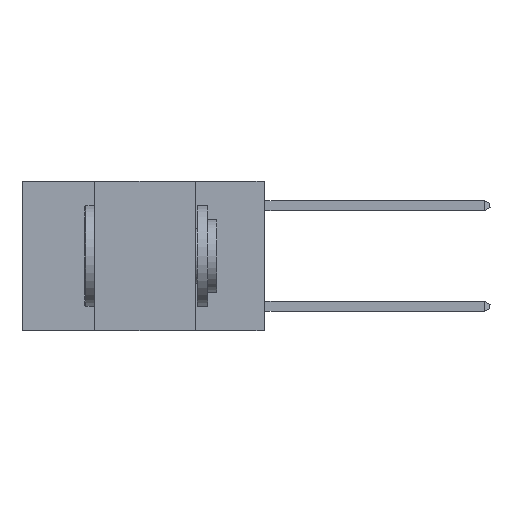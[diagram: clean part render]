
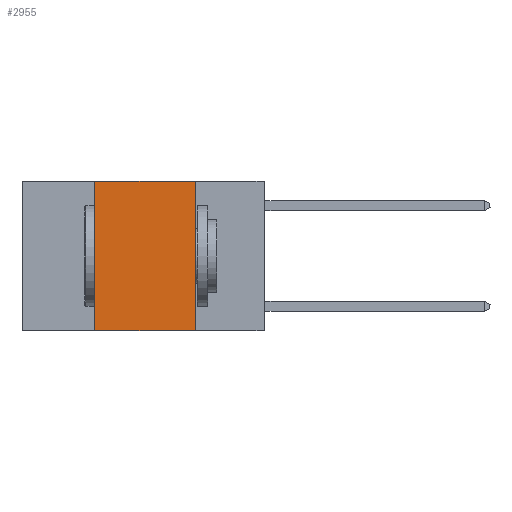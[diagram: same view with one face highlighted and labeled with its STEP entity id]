
A CAD part, left-side view. The second image highlights one B-rep face of the part: STEP entity #2955.
In plain terms, the highlighted planar face has unit normal (-1, 0, 0).
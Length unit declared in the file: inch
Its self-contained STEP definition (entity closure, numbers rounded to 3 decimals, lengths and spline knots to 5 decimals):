
#1292 = ORIENTED_EDGE ( 'NONE', *, *, #1631, .T. ) ;
#1631 = EDGE_CURVE ( 'NONE', #12407, #27223, #18043, .T. ) ;
#1664 = CARTESIAN_POINT ( 'NONE',  ( 0., 0.17, -0.37 ) ) ;
#2785 = ORIENTED_EDGE ( 'NONE', *, *, #22807, .F. ) ;
#2955 = ADVANCED_FACE ( 'NONE', ( #5064 ), #23852, .F. ) ;
#3249 = CARTESIAN_POINT ( 'NONE',  ( 0., 0.42, 0. ) ) ;
#3257 = LINE ( 'NONE', #19297, #18643 ) ;
#3415 = ORIENTED_EDGE ( 'NONE', *, *, #21486, .F. ) ;
#4548 = VERTEX_POINT ( 'NONE', #15883 ) ;
#4692 = CARTESIAN_POINT ( 'NONE',  ( 0., 0.6, 0. ) ) ;
#5050 = EDGE_CURVE ( 'NONE', #4548, #10568, #18582, .T. ) ;
#5064 = FACE_OUTER_BOUND ( 'NONE', #8661, .T. ) ;
#5957 = VECTOR ( 'NONE', #13002, 39.37008 ) ;
#6549 = DIRECTION ( 'NONE',  ( 0., -1., 0. ) ) ;
#7078 = ORIENTED_EDGE ( 'NONE', *, *, #5050, .F. ) ;
#8661 = EDGE_LOOP ( 'NONE', ( #2785, #7078, #3415, #1292 ) ) ;
#10568 = VERTEX_POINT ( 'NONE', #19948 ) ;
#11600 = VECTOR ( 'NONE', #12578, 39.37008 ) ;
#12226 = DIRECTION ( 'NONE',  ( 1., 0., 0. ) ) ;
#12407 = VERTEX_POINT ( 'NONE', #21195 ) ;
#12578 = DIRECTION ( 'NONE',  ( 0., 0., 1. ) ) ;
#13002 = DIRECTION ( 'NONE',  ( 0., -1., 0. ) ) ;
#13422 = AXIS2_PLACEMENT_3D ( 'NONE', #23538, #12226, #18946 ) ;
#15883 = CARTESIAN_POINT ( 'NONE',  ( 0., 0.42, 0. ) ) ;
#18043 = LINE ( 'NONE', #22158, #5957 ) ;
#18582 = LINE ( 'NONE', #4692, #25816 ) ;
#18643 = VECTOR ( 'NONE', #28647, 39.37008 ) ;
#18946 = DIRECTION ( 'NONE',  ( 0., 0., -1. ) ) ;
#19297 = CARTESIAN_POINT ( 'NONE',  ( 0., 0.17, 0. ) ) ;
#19948 = CARTESIAN_POINT ( 'NONE',  ( 0., 0.17, 0. ) ) ;
#21195 = CARTESIAN_POINT ( 'NONE',  ( 0., 0.42, -0.37 ) ) ;
#21486 = EDGE_CURVE ( 'NONE', #12407, #4548, #26650, .T. ) ;
#22158 = CARTESIAN_POINT ( 'NONE',  ( 0., 0.6, -0.37 ) ) ;
#22807 = EDGE_CURVE ( 'NONE', #10568, #27223, #3257, .T. ) ;
#23538 = CARTESIAN_POINT ( 'NONE',  ( 0., 0.6, 0. ) ) ;
#23852 = PLANE ( 'NONE',  #13422 ) ;
#25816 = VECTOR ( 'NONE', #6549, 39.37008 ) ;
#26650 = LINE ( 'NONE', #3249, #11600 ) ;
#27223 = VERTEX_POINT ( 'NONE', #1664 ) ;
#28647 = DIRECTION ( 'NONE',  ( 0., 0., -1. ) ) ;
